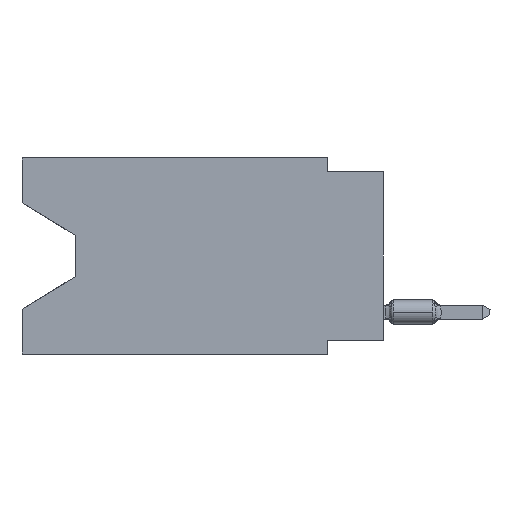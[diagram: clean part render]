
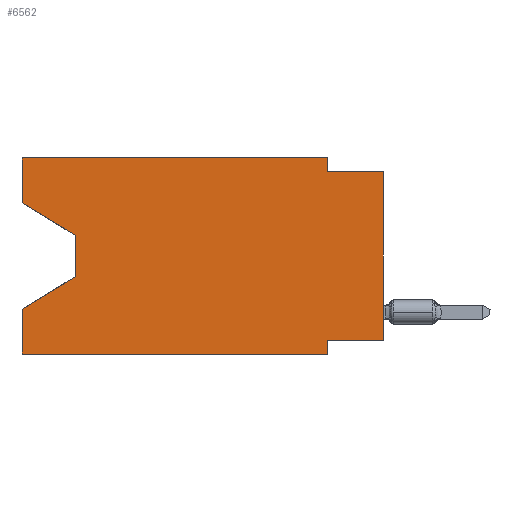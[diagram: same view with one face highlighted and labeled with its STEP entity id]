
A CAD part, left-side view. The second image highlights one B-rep face of the part: STEP entity #6562.
In plain terms, the highlighted planar face has unit normal (-1, 0, 0).
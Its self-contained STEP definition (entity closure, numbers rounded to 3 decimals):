
#139 = VERTEX_POINT ( 'NONE', #21280 ) ;
#548 = EDGE_CURVE ( 'NONE', #25592, #27506, #14798, .T. ) ;
#675 = EDGE_CURVE ( 'NONE', #27506, #6577, #22648, .T. ) ;
#809 = VERTEX_POINT ( 'NONE', #21494 ) ;
#987 = DIRECTION ( 'NONE',  ( 0., 0., 1. ) ) ;
#1329 = DIRECTION ( 'NONE',  ( 0., -0.855, -0.519 ) ) ;
#1756 = EDGE_CURVE ( 'NONE', #809, #14532, #2878, .T. ) ;
#1781 = DIRECTION ( 'NONE',  ( 0., 0., -1. ) ) ;
#2170 = EDGE_CURVE ( 'NONE', #26873, #139, #23164, .T. ) ;
#2878 = LINE ( 'NONE', #16057, #26841 ) ;
#3185 = CARTESIAN_POINT ( 'NONE',  ( 0., 0., 0. ) ) ;
#3849 = VECTOR ( 'NONE', #1329, 1000. ) ;
#4110 = DIRECTION ( 'NONE',  ( 0., -1., 0. ) ) ;
#4762 = CARTESIAN_POINT ( 'NONE',  ( 0., 13.97, -5.385 ) ) ;
#4795 = DIRECTION ( 'NONE',  ( 0., -1., 0. ) ) ;
#4848 = AXIS2_PLACEMENT_3D ( 'NONE', #22622, #27150, #9293 ) ;
#4887 = ORIENTED_EDGE ( 'NONE', *, *, #21771, .F. ) ;
#5169 = DIRECTION ( 'NONE',  ( 0., 0., 1. ) ) ;
#5317 = EDGE_CURVE ( 'NONE', #6577, #139, #28576, .T. ) ;
#5485 = LINE ( 'NONE', #21143, #9763 ) ;
#5495 = VERTEX_POINT ( 'NONE', #10849 ) ;
#5635 = DIRECTION ( 'NONE',  ( 0., 1., 0. ) ) ;
#6036 = DIRECTION ( 'NONE',  ( 0., 0.855, -0.519 ) ) ;
#6562 = ADVANCED_FACE ( 'NONE', ( #18668 ), #24957, .F. ) ;
#6577 = VERTEX_POINT ( 'NONE', #4762 ) ;
#7700 = ORIENTED_EDGE ( 'NONE', *, *, #8029, .F. ) ;
#8029 = EDGE_CURVE ( 'NONE', #25592, #809, #15142, .T. ) ;
#9173 = CARTESIAN_POINT ( 'NONE',  ( 0., 13.97, -3.505 ) ) ;
#9293 = DIRECTION ( 'NONE',  ( 0., 0., -1. ) ) ;
#9660 = ORIENTED_EDGE ( 'NONE', *, *, #16149, .T. ) ;
#9763 = VECTOR ( 'NONE', #5635, 1000. ) ;
#9911 = CARTESIAN_POINT ( 'NONE',  ( 0., 16.383, -8.89 ) ) ;
#9927 = CARTESIAN_POINT ( 'NONE',  ( 0., 0., -0.635 ) ) ;
#10645 = EDGE_CURVE ( 'NONE', #5495, #17917, #27785, .T. ) ;
#10849 = CARTESIAN_POINT ( 'NONE',  ( 0., 0., -8.255 ) ) ;
#10872 = EDGE_LOOP ( 'NONE', ( #17270, #26065, #12964, #28904, #9660, #15120, #23135, #18284, #4887, #12298, #19177, #7700 ) ) ;
#10984 = CARTESIAN_POINT ( 'NONE',  ( 0., 2.54, 0. ) ) ;
#11816 = VECTOR ( 'NONE', #6036, 1000. ) ;
#12146 = VECTOR ( 'NONE', #17401, 1000. ) ;
#12298 = ORIENTED_EDGE ( 'NONE', *, *, #21571, .F. ) ;
#12964 = ORIENTED_EDGE ( 'NONE', *, *, #5317, .T. ) ;
#13669 = EDGE_CURVE ( 'NONE', #24862, #19800, #23855, .T. ) ;
#14532 = VERTEX_POINT ( 'NONE', #19504 ) ;
#14798 = LINE ( 'NONE', #21391, #3849 ) ;
#15120 = ORIENTED_EDGE ( 'NONE', *, *, #13669, .F. ) ;
#15142 = LINE ( 'NONE', #22317, #19823 ) ;
#15500 = LINE ( 'NONE', #24440, #26216 ) ;
#16017 = CARTESIAN_POINT ( 'NONE',  ( 0., 2.54, -0.635 ) ) ;
#16057 = CARTESIAN_POINT ( 'NONE',  ( 0., 16.383, 0. ) ) ;
#16149 = EDGE_CURVE ( 'NONE', #26873, #19800, #15500, .T. ) ;
#16384 = LINE ( 'NONE', #9927, #19493 ) ;
#16574 = CARTESIAN_POINT ( 'NONE',  ( 0., 16.383, 0. ) ) ;
#17270 = ORIENTED_EDGE ( 'NONE', *, *, #548, .T. ) ;
#17401 = DIRECTION ( 'NONE',  ( 0., 0., -1. ) ) ;
#17917 = VERTEX_POINT ( 'NONE', #27280 ) ;
#18284 = ORIENTED_EDGE ( 'NONE', *, *, #10645, .T. ) ;
#18668 = FACE_OUTER_BOUND ( 'NONE', #10872, .T. ) ;
#18879 = DIRECTION ( 'NONE',  ( 0., -1., 0. ) ) ;
#19177 = ORIENTED_EDGE ( 'NONE', *, *, #1756, .F. ) ;
#19319 = VECTOR ( 'NONE', #5169, 1000. ) ;
#19493 = VECTOR ( 'NONE', #18879, 1000. ) ;
#19504 = CARTESIAN_POINT ( 'NONE',  ( 0., 2.54, 0. ) ) ;
#19658 = CARTESIAN_POINT ( 'NONE',  ( 0., 13.97, -5.385 ) ) ;
#19800 = VERTEX_POINT ( 'NONE', #27554 ) ;
#19823 = VECTOR ( 'NONE', #24506, 1000. ) ;
#20828 = CARTESIAN_POINT ( 'NONE',  ( 0., 2.54, -8.255 ) ) ;
#21143 = CARTESIAN_POINT ( 'NONE',  ( 0., 0., -8.255 ) ) ;
#21280 = CARTESIAN_POINT ( 'NONE',  ( 0., 16.383, -6.852 ) ) ;
#21391 = CARTESIAN_POINT ( 'NONE',  ( 0., 16.383, -2.038 ) ) ;
#21494 = CARTESIAN_POINT ( 'NONE',  ( 0., 16.383, 0. ) ) ;
#21571 = EDGE_CURVE ( 'NONE', #14532, #23660, #26651, .T. ) ;
#21771 = EDGE_CURVE ( 'NONE', #23660, #17917, #16384, .T. ) ;
#22094 = VECTOR ( 'NONE', #28564, 1000. ) ;
#22317 = CARTESIAN_POINT ( 'NONE',  ( 0., 16.383, 0. ) ) ;
#22622 = CARTESIAN_POINT ( 'NONE',  ( 0., 16.383, 0. ) ) ;
#22648 = LINE ( 'NONE', #9173, #22094 ) ;
#22727 = VECTOR ( 'NONE', #1781, 1000. ) ;
#23135 = ORIENTED_EDGE ( 'NONE', *, *, #23810, .F. ) ;
#23164 = LINE ( 'NONE', #16574, #19319 ) ;
#23660 = VERTEX_POINT ( 'NONE', #16017 ) ;
#23704 = CARTESIAN_POINT ( 'NONE',  ( 0., 2.54, -8.89 ) ) ;
#23810 = EDGE_CURVE ( 'NONE', #5495, #24862, #5485, .T. ) ;
#23855 = LINE ( 'NONE', #23704, #12146 ) ;
#24440 = CARTESIAN_POINT ( 'NONE',  ( 0., 16.383, -8.89 ) ) ;
#24506 = DIRECTION ( 'NONE',  ( 0., 0., 1. ) ) ;
#24862 = VERTEX_POINT ( 'NONE', #20828 ) ;
#24957 = PLANE ( 'NONE',  #4848 ) ;
#25592 = VERTEX_POINT ( 'NONE', #26631 ) ;
#26065 = ORIENTED_EDGE ( 'NONE', *, *, #675, .T. ) ;
#26216 = VECTOR ( 'NONE', #4110, 1000. ) ;
#26631 = CARTESIAN_POINT ( 'NONE',  ( 0., 16.383, -2.038 ) ) ;
#26651 = LINE ( 'NONE', #10984, #22727 ) ;
#26841 = VECTOR ( 'NONE', #4795, 1000. ) ;
#26873 = VERTEX_POINT ( 'NONE', #9911 ) ;
#27150 = DIRECTION ( 'NONE',  ( 1., 0., 0. ) ) ;
#27280 = CARTESIAN_POINT ( 'NONE',  ( 0., 0., -0.635 ) ) ;
#27384 = VECTOR ( 'NONE', #987, 1000. ) ;
#27405 = CARTESIAN_POINT ( 'NONE',  ( 0., 13.97, -3.505 ) ) ;
#27506 = VERTEX_POINT ( 'NONE', #27405 ) ;
#27554 = CARTESIAN_POINT ( 'NONE',  ( 0., 2.54, -8.89 ) ) ;
#27785 = LINE ( 'NONE', #3185, #27384 ) ;
#28564 = DIRECTION ( 'NONE',  ( 0., 0., -1. ) ) ;
#28576 = LINE ( 'NONE', #19658, #11816 ) ;
#28904 = ORIENTED_EDGE ( 'NONE', *, *, #2170, .F. ) ;
